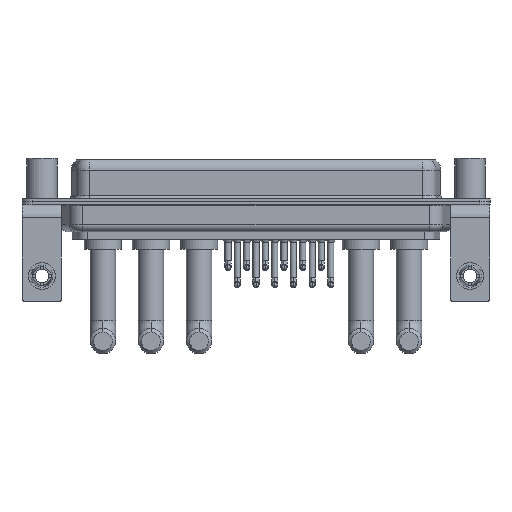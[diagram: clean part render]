
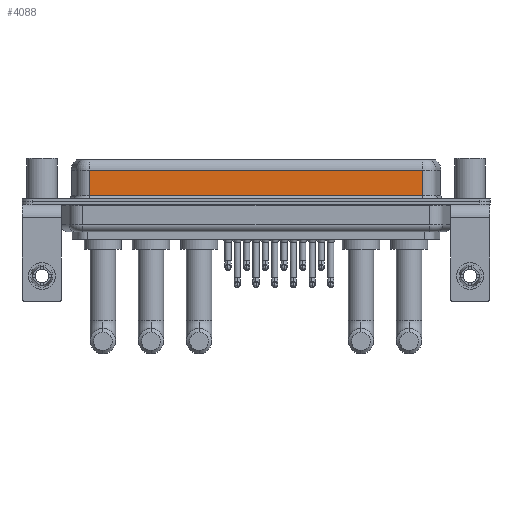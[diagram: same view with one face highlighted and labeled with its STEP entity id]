
A CAD part, front view. The second image highlights one B-rep face of the part: STEP entity #4088.
In plain terms, the highlighted planar face has unit normal (0, -1, 0).
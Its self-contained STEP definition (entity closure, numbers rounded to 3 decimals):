
#435 = ORIENTED_EDGE ( 'NONE', *, *, #14255, .T. ) ;
#862 = PLANE ( 'NONE',  #15004 ) ;
#3652 = EDGE_LOOP ( 'NONE', ( #4379, #435, #15316, #21616 ) ) ;
#4088 = ADVANCED_FACE ( 'NONE', ( #5071 ), #862, .F. ) ;
#4379 = ORIENTED_EDGE ( 'NONE', *, *, #10166, .F. ) ;
#5011 = LINE ( 'NONE', #19681, #6124 ) ;
#5071 = FACE_OUTER_BOUND ( 'NONE', #3652, .T. ) ;
#6124 = VECTOR ( 'NONE', #18185, 1000. ) ;
#7489 = VERTEX_POINT ( 'NONE', #19396 ) ;
#9476 = VERTEX_POINT ( 'NONE', #17400 ) ;
#10166 = EDGE_CURVE ( 'NONE', #10769, #7489, #5011, .T. ) ;
#10769 = VERTEX_POINT ( 'NONE', #14576 ) ;
#12557 = DIRECTION ( 'NONE',  ( 0., 1., 0. ) ) ;
#13323 = CARTESIAN_POINT ( 'NONE',  ( 7.038, -3.95, 4.65 ) ) ;
#14255 = EDGE_CURVE ( 'NONE', #10769, #14402, #24210, .T. ) ;
#14402 = VERTEX_POINT ( 'NONE', #13323 ) ;
#14406 = DIRECTION ( 'NONE',  ( 1., 0., 0. ) ) ;
#14576 = CARTESIAN_POINT ( 'NONE',  ( 56.462, -3.95, 4.65 ) ) ;
#14862 = VECTOR ( 'NONE', #23941, 1000. ) ;
#15004 = AXIS2_PLACEMENT_3D ( 'NONE', #17876, #12557, #19606 ) ;
#15316 = ORIENTED_EDGE ( 'NONE', *, *, #18473, .T. ) ;
#16551 = LINE ( 'NONE', #24188, #14862 ) ;
#17400 = CARTESIAN_POINT ( 'NONE',  ( 7.038, -3.95, 0.9 ) ) ;
#17876 = CARTESIAN_POINT ( 'NONE',  ( 56.462, -3.95, 6.4 ) ) ;
#18185 = DIRECTION ( 'NONE',  ( 0., 0., -1. ) ) ;
#18473 = EDGE_CURVE ( 'NONE', #14402, #9476, #16551, .T. ) ;
#19396 = CARTESIAN_POINT ( 'NONE',  ( 56.462, -3.95, 0.9 ) ) ;
#19606 = DIRECTION ( 'NONE',  ( 0., 0., 1. ) ) ;
#19681 = CARTESIAN_POINT ( 'NONE',  ( 56.462, -3.95, 6.4 ) ) ;
#20278 = CARTESIAN_POINT ( 'NONE',  ( 56.462, -3.95, 4.65 ) ) ;
#20549 = VECTOR ( 'NONE', #14406, 1000. ) ;
#21616 = ORIENTED_EDGE ( 'NONE', *, *, #23976, .T. ) ;
#22243 = DIRECTION ( 'NONE',  ( -1., 0., 0. ) ) ;
#23941 = DIRECTION ( 'NONE',  ( 0., 0., -1. ) ) ;
#23976 = EDGE_CURVE ( 'NONE', #9476, #7489, #24162, .T. ) ;
#24162 = LINE ( 'NONE', #24281, #20549 ) ;
#24188 = CARTESIAN_POINT ( 'NONE',  ( 7.038, -3.95, 6.4 ) ) ;
#24210 = LINE ( 'NONE', #20278, #24341 ) ;
#24281 = CARTESIAN_POINT ( 'NONE',  ( 56.462, -3.95, 0.9 ) ) ;
#24341 = VECTOR ( 'NONE', #22243, 1000. ) ;
